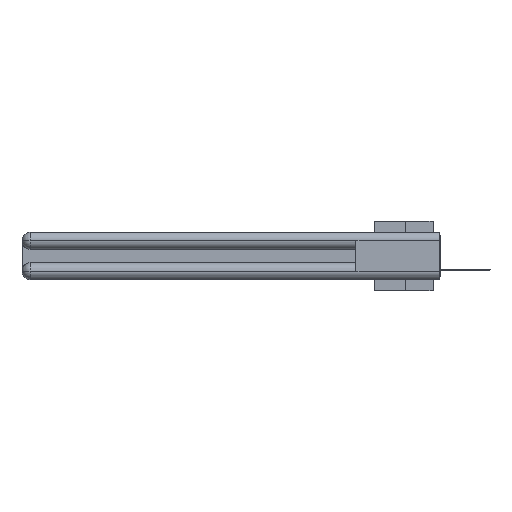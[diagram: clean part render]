
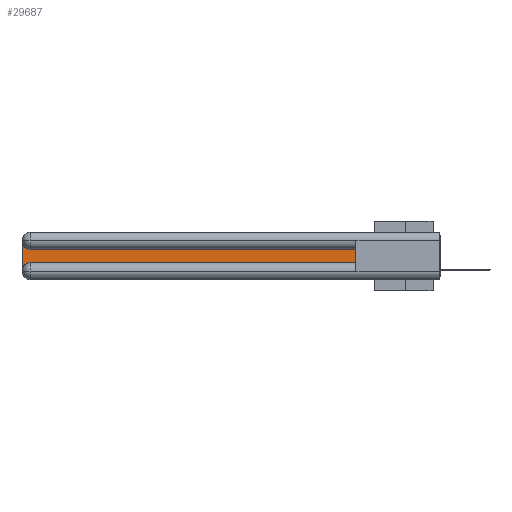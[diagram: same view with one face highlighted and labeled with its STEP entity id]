
A CAD part, left-side view. The second image highlights one B-rep face of the part: STEP entity #29687.
In plain terms, the highlighted planar face has unit normal (-1, 0, 0).
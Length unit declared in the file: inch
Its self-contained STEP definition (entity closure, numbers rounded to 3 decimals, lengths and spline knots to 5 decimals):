
#731 = DIRECTION ( 'NONE',  ( 1., 0., 0. ) ) ;
#1771 = EDGE_CURVE ( 'NONE', #5707, #26214, #11856, .T. ) ;
#1878 = LINE ( 'NONE', #6146, #9459 ) ;
#1906 = ORIENTED_EDGE ( 'NONE', *, *, #1771, .T. ) ;
#2691 = VERTEX_POINT ( 'NONE', #18074 ) ;
#3342 = DIRECTION ( 'NONE',  ( 0., 0., -1. ) ) ;
#3484 = EDGE_CURVE ( 'NONE', #14869, #5707, #6122, .T. ) ;
#3777 = EDGE_CURVE ( 'NONE', #15612, #14869, #19758, .T. ) ;
#5707 = VERTEX_POINT ( 'NONE', #25485 ) ;
#5795 = CARTESIAN_POINT ( 'NONE',  ( 0.075, 0.6, -0.2175 ) ) ;
#6122 = CIRCLE ( 'NONE', #28746, 0.06 ) ;
#6146 = CARTESIAN_POINT ( 'NONE',  ( 0.075, 0.6, -0.1225 ) ) ;
#6801 = DIRECTION ( 'NONE',  ( 0., 0., -1. ) ) ;
#6921 = DIRECTION ( 'NONE',  ( 1., 0., 0. ) ) ;
#8924 = VECTOR ( 'NONE', #11695, 39.37008 ) ;
#9183 = DIRECTION ( 'NONE',  ( 0., 0., -1. ) ) ;
#9459 = VECTOR ( 'NONE', #15333, 39.37008 ) ;
#9607 = CARTESIAN_POINT ( 'NONE',  ( 0.075, 0.6, -0.2175 ) ) ;
#9672 = CARTESIAN_POINT ( 'NONE',  ( 0.075, 3., -0.1225 ) ) ;
#10628 = CARTESIAN_POINT ( 'NONE',  ( 0.075, 3., -0.2775 ) ) ;
#11173 = DIRECTION ( 'NONE',  ( 1., 0., 0. ) ) ;
#11523 = ORIENTED_EDGE ( 'NONE', *, *, #3484, .T. ) ;
#11650 = VECTOR ( 'NONE', #12713, 39.37008 ) ;
#11695 = DIRECTION ( 'NONE',  ( 0., -1., 0. ) ) ;
#11856 = LINE ( 'NONE', #9607, #8924 ) ;
#12713 = DIRECTION ( 'NONE',  ( 0., 0., 1. ) ) ;
#14005 = CARTESIAN_POINT ( 'NONE',  ( 0.075, 2.94, -0.0625 ) ) ;
#14521 = LINE ( 'NONE', #5795, #11650 ) ;
#14869 = VERTEX_POINT ( 'NONE', #10628 ) ;
#14935 = AXIS2_PLACEMENT_3D ( 'NONE', #14005, #6921, #9183 ) ;
#15037 = CARTESIAN_POINT ( 'NONE',  ( 0.075, 0.6, -0.1225 ) ) ;
#15333 = DIRECTION ( 'NONE',  ( 0., 1., 0. ) ) ;
#15612 = VERTEX_POINT ( 'NONE', #17774 ) ;
#16482 = ORIENTED_EDGE ( 'NONE', *, *, #19007, .T. ) ;
#16680 = AXIS2_PLACEMENT_3D ( 'NONE', #9672, #731, #19446 ) ;
#17774 = CARTESIAN_POINT ( 'NONE',  ( 0.075, 3., -0.0625 ) ) ;
#18074 = CARTESIAN_POINT ( 'NONE',  ( 0.075, 2.94, -0.1225 ) ) ;
#18154 = VECTOR ( 'NONE', #3342, 39.37008 ) ;
#19007 = EDGE_CURVE ( 'NONE', #21656, #2691, #1878, .T. ) ;
#19309 = CARTESIAN_POINT ( 'NONE',  ( 0.075, 3., -0.2175 ) ) ;
#19446 = DIRECTION ( 'NONE',  ( 0., 0., -1. ) ) ;
#19758 = LINE ( 'NONE', #19309, #18154 ) ;
#21656 = VERTEX_POINT ( 'NONE', #15037 ) ;
#23179 = EDGE_CURVE ( 'NONE', #2691, #15612, #27927, .T. ) ;
#23288 = ORIENTED_EDGE ( 'NONE', *, *, #3777, .T. ) ;
#23369 = FACE_OUTER_BOUND ( 'NONE', #25564, .T. ) ;
#23849 = EDGE_CURVE ( 'NONE', #26214, #21656, #14521, .T. ) ;
#25485 = CARTESIAN_POINT ( 'NONE',  ( 0.075, 2.94, -0.2175 ) ) ;
#25564 = EDGE_LOOP ( 'NONE', ( #16482, #29321, #23288, #11523, #1906, #29657 ) ) ;
#26062 = PLANE ( 'NONE',  #16680 ) ;
#26214 = VERTEX_POINT ( 'NONE', #26337 ) ;
#26337 = CARTESIAN_POINT ( 'NONE',  ( 0.075, 0.6, -0.2175 ) ) ;
#27445 = CARTESIAN_POINT ( 'NONE',  ( 0.075, 2.94, -0.2775 ) ) ;
#27927 = CIRCLE ( 'NONE', #14935, 0.06 ) ;
#28746 = AXIS2_PLACEMENT_3D ( 'NONE', #27445, #11173, #6801 ) ;
#29321 = ORIENTED_EDGE ( 'NONE', *, *, #23179, .T. ) ;
#29657 = ORIENTED_EDGE ( 'NONE', *, *, #23849, .T. ) ;
#29687 = ADVANCED_FACE ( 'NONE', ( #23369 ), #26062, .F. ) ;
